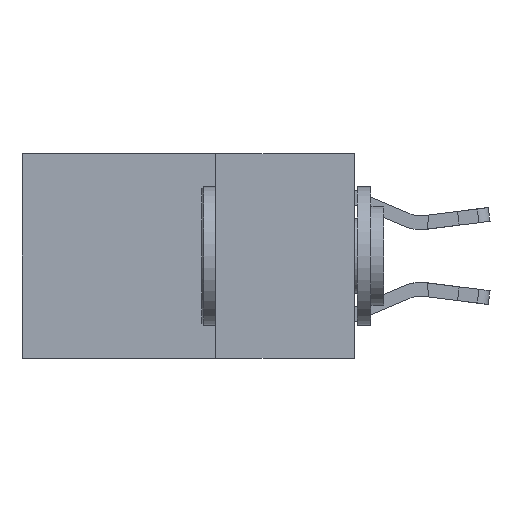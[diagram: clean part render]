
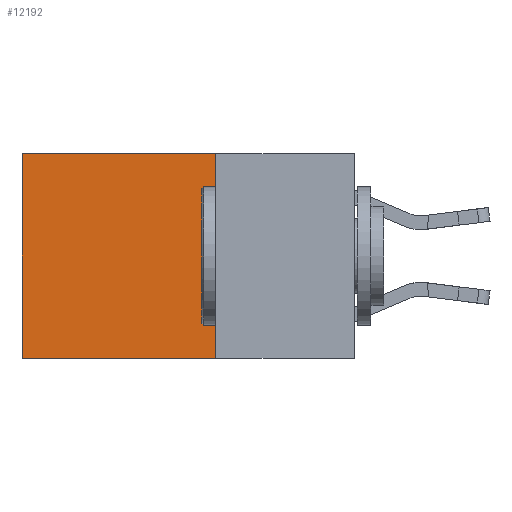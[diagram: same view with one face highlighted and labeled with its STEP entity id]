
A CAD part, left-side view. The second image highlights one B-rep face of the part: STEP entity #12192.
In plain terms, the highlighted planar face has unit normal (-1, 0, 0).
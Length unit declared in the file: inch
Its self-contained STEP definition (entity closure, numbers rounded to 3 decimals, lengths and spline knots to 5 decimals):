
#236 = LINE ( 'NONE', #1473, #11342 ) ;
#367 = DIRECTION ( 'NONE',  ( 0., 0., -1. ) ) ;
#487 = VERTEX_POINT ( 'NONE', #9195 ) ;
#1473 = CARTESIAN_POINT ( 'NONE',  ( 0.2625, 0.6, 0. ) ) ;
#1632 = AXIS2_PLACEMENT_3D ( 'NONE', #7374, #13414, #12196 ) ;
#2073 = ORIENTED_EDGE ( 'NONE', *, *, #8877, .F. ) ;
#2654 = ORIENTED_EDGE ( 'NONE', *, *, #9537, .T. ) ;
#3949 = DIRECTION ( 'NONE',  ( 0., 1., 0. ) ) ;
#4009 = CARTESIAN_POINT ( 'NONE',  ( 0.2625, 0.6, 0. ) ) ;
#4883 = EDGE_LOOP ( 'NONE', ( #15269, #10519, #2073, #2654 ) ) ;
#5010 = LINE ( 'NONE', #7419, #8863 ) ;
#5667 = DIRECTION ( 'NONE',  ( 0., 0., -1. ) ) ;
#7374 = CARTESIAN_POINT ( 'NONE',  ( 0.2625, 0.25, 0. ) ) ;
#7419 = CARTESIAN_POINT ( 'NONE',  ( 0.2625, 0.25, 0. ) ) ;
#7450 = PLANE ( 'NONE',  #1632 ) ;
#7621 = LINE ( 'NONE', #15214, #13371 ) ;
#8863 = VECTOR ( 'NONE', #12237, 39.37008 ) ;
#8877 = EDGE_CURVE ( 'NONE', #13584, #9026, #7621, .T. ) ;
#9026 = VERTEX_POINT ( 'NONE', #11163 ) ;
#9195 = CARTESIAN_POINT ( 'NONE',  ( 0.2625, 0.6, -0.37 ) ) ;
#9537 = EDGE_CURVE ( 'NONE', #13584, #12107, #5010, .T. ) ;
#9787 = CARTESIAN_POINT ( 'NONE',  ( 0.2625, 0.25, -0.37 ) ) ;
#10414 = EDGE_CURVE ( 'NONE', #12107, #487, #236, .T. ) ;
#10519 = ORIENTED_EDGE ( 'NONE', *, *, #14292, .F. ) ;
#11163 = CARTESIAN_POINT ( 'NONE',  ( 0.2625, 0.25, -0.37 ) ) ;
#11342 = VECTOR ( 'NONE', #367, 39.37008 ) ;
#12107 = VERTEX_POINT ( 'NONE', #4009 ) ;
#12192 = ADVANCED_FACE ( 'NONE', ( #13193 ), #7450, .F. ) ;
#12196 = DIRECTION ( 'NONE',  ( 0., 0., -1. ) ) ;
#12237 = DIRECTION ( 'NONE',  ( 0., 1., 0. ) ) ;
#13193 = FACE_OUTER_BOUND ( 'NONE', #4883, .T. ) ;
#13371 = VECTOR ( 'NONE', #5667, 39.37008 ) ;
#13414 = DIRECTION ( 'NONE',  ( 1., 0., 0. ) ) ;
#13584 = VERTEX_POINT ( 'NONE', #14823 ) ;
#14292 = EDGE_CURVE ( 'NONE', #9026, #487, #14615, .T. ) ;
#14339 = VECTOR ( 'NONE', #3949, 39.37008 ) ;
#14615 = LINE ( 'NONE', #9787, #14339 ) ;
#14823 = CARTESIAN_POINT ( 'NONE',  ( 0.2625, 0.25, 0. ) ) ;
#15214 = CARTESIAN_POINT ( 'NONE',  ( 0.2625, 0.25, 0. ) ) ;
#15269 = ORIENTED_EDGE ( 'NONE', *, *, #10414, .T. ) ;
